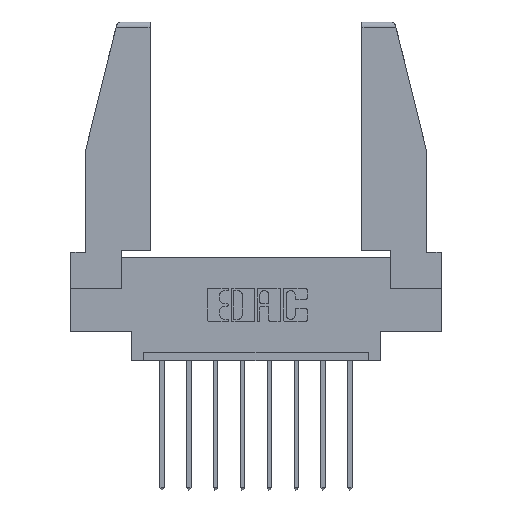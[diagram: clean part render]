
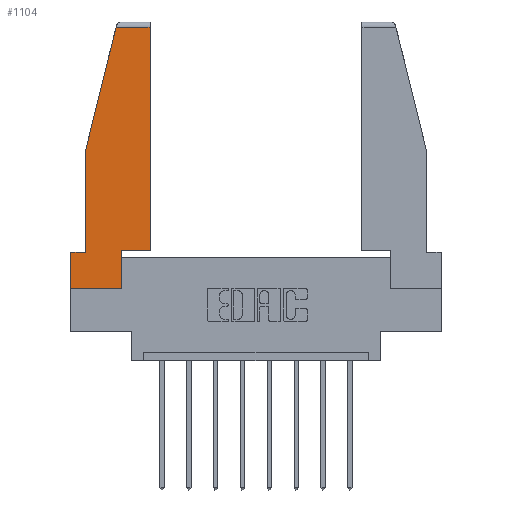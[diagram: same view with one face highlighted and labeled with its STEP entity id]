
A CAD part, top view. The second image highlights one B-rep face of the part: STEP entity #1104.
In plain terms, the highlighted planar face has unit normal (0, 0, 1).
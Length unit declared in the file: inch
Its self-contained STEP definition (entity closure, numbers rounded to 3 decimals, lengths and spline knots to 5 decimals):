
#374 = ORIENTED_EDGE ( 'NONE', *, *, #4284, .T. ) ;
#571 = CARTESIAN_POINT ( 'NONE',  ( 0.297, 0., 0. ) ) ;
#787 = VERTEX_POINT ( 'NONE', #571 ) ;
#993 = CARTESIAN_POINT ( 'NONE',  ( 0.086, 0.21, 0. ) ) ;
#1021 = VERTEX_POINT ( 'NONE', #4981 ) ;
#1044 = CARTESIAN_POINT ( 'NONE',  ( 0.297, 0.223, 0. ) ) ;
#1104 = ADVANCED_FACE ( 'NONE', ( #7009 ), #9016, .T. ) ;
#1196 = DIRECTION ( 'NONE',  ( 1., 0., 0. ) ) ;
#1366 = VERTEX_POINT ( 'NONE', #2493 ) ;
#1402 = EDGE_CURVE ( 'NONE', #1366, #1021, #10311, .T. ) ;
#1711 = ORIENTED_EDGE ( 'NONE', *, *, #8019, .T. ) ;
#1864 = LINE ( 'NONE', #9884, #8875 ) ;
#2055 = CARTESIAN_POINT ( 'NONE',  ( 0.297, 0.223, 0. ) ) ;
#2300 = LINE ( 'NONE', #12839, #4315 ) ;
#2321 = VECTOR ( 'NONE', #5635, 39.37008 ) ;
#2493 = CARTESIAN_POINT ( 'NONE',  ( 0.461, 1.52, 0. ) ) ;
#2699 = CARTESIAN_POINT ( 'NONE',  ( 0., 1.52, 0. ) ) ;
#2804 = LINE ( 'NONE', #8378, #10902 ) ;
#3089 = DIRECTION ( 'NONE',  ( 0., 0., 1. ) ) ;
#3098 = ORIENTED_EDGE ( 'NONE', *, *, #11533, .T. ) ;
#3174 = DIRECTION ( 'NONE',  ( -0.239, -0.971, 0. ) ) ;
#3208 = CARTESIAN_POINT ( 'NONE',  ( 0., 0., 0. ) ) ;
#3482 = VECTOR ( 'NONE', #10909, 39.37008 ) ;
#3798 = CARTESIAN_POINT ( 'NONE',  ( 0.086, 0.8, 0. ) ) ;
#3975 = LINE ( 'NONE', #8621, #11837 ) ;
#4070 = CARTESIAN_POINT ( 'NONE',  ( 0., 0., 0. ) ) ;
#4145 = CARTESIAN_POINT ( 'NONE',  ( 0., 0.21, 0. ) ) ;
#4284 = EDGE_CURVE ( 'NONE', #11437, #12099, #7733, .T. ) ;
#4315 = VECTOR ( 'NONE', #11836, 39.37008 ) ;
#4981 = CARTESIAN_POINT ( 'NONE',  ( 0.2636, 1.52, 0. ) ) ;
#5076 = ORIENTED_EDGE ( 'NONE', *, *, #8603, .T. ) ;
#5110 = ORIENTED_EDGE ( 'NONE', *, *, #1402, .T. ) ;
#5635 = DIRECTION ( 'NONE',  ( -1., 0., 0. ) ) ;
#5682 = EDGE_CURVE ( 'NONE', #11291, #787, #7548, .T. ) ;
#5814 = LINE ( 'NONE', #9106, #8008 ) ;
#5994 = VECTOR ( 'NONE', #11102, 39.37008 ) ;
#6063 = EDGE_CURVE ( 'NONE', #787, #7178, #5814, .T. ) ;
#6149 = EDGE_CURVE ( 'NONE', #7178, #9299, #7037, .T. ) ;
#6371 = ORIENTED_EDGE ( 'NONE', *, *, #6063, .T. ) ;
#6395 = CARTESIAN_POINT ( 'NONE',  ( 0.461, 0.223, 0. ) ) ;
#6907 = DIRECTION ( 'NONE',  ( 0., 1., 0. ) ) ;
#7009 = FACE_OUTER_BOUND ( 'NONE', #10683, .T. ) ;
#7037 = LINE ( 'NONE', #1044, #12554 ) ;
#7149 = CARTESIAN_POINT ( 'NONE',  ( 0.086, 0.8, 0. ) ) ;
#7178 = VERTEX_POINT ( 'NONE', #2055 ) ;
#7278 = ORIENTED_EDGE ( 'NONE', *, *, #9444, .T. ) ;
#7437 = VERTEX_POINT ( 'NONE', #4145 ) ;
#7548 = LINE ( 'NONE', #4070, #5994 ) ;
#7733 = LINE ( 'NONE', #3798, #3482 ) ;
#8008 = VECTOR ( 'NONE', #6907, 39.37008 ) ;
#8019 = EDGE_CURVE ( 'NONE', #1021, #11437, #1864, .T. ) ;
#8378 = CARTESIAN_POINT ( 'NONE',  ( 0., 0.21, 0. ) ) ;
#8603 = EDGE_CURVE ( 'NONE', #9299, #1366, #2300, .T. ) ;
#8621 = CARTESIAN_POINT ( 'NONE',  ( 0., 0.21, 0. ) ) ;
#8875 = VECTOR ( 'NONE', #3174, 39.37008 ) ;
#9016 = PLANE ( 'NONE',  #11665 ) ;
#9106 = CARTESIAN_POINT ( 'NONE',  ( 0.297, 0., 0. ) ) ;
#9299 = VERTEX_POINT ( 'NONE', #6395 ) ;
#9443 = DIRECTION ( 'NONE',  ( 0., -1., 0. ) ) ;
#9444 = EDGE_CURVE ( 'NONE', #12099, #7437, #3975, .T. ) ;
#9686 = DIRECTION ( 'NONE',  ( -1., 0., 0. ) ) ;
#9884 = CARTESIAN_POINT ( 'NONE',  ( 0.271, 1.55, 0. ) ) ;
#10311 = LINE ( 'NONE', #2699, #2321 ) ;
#10683 = EDGE_LOOP ( 'NONE', ( #5076, #5110, #1711, #374, #7278, #3098, #11795, #6371, #12074 ) ) ;
#10902 = VECTOR ( 'NONE', #9443, 39.37008 ) ;
#10909 = DIRECTION ( 'NONE',  ( 0., -1., 0. ) ) ;
#11091 = CARTESIAN_POINT ( 'NONE',  ( 0., 0., 0. ) ) ;
#11102 = DIRECTION ( 'NONE',  ( 1., 0., 0. ) ) ;
#11291 = VERTEX_POINT ( 'NONE', #3208 ) ;
#11437 = VERTEX_POINT ( 'NONE', #7149 ) ;
#11533 = EDGE_CURVE ( 'NONE', #7437, #11291, #2804, .T. ) ;
#11665 = AXIS2_PLACEMENT_3D ( 'NONE', #11091, #3089, #1196 ) ;
#11795 = ORIENTED_EDGE ( 'NONE', *, *, #5682, .T. ) ;
#11836 = DIRECTION ( 'NONE',  ( 0., 1., 0. ) ) ;
#11837 = VECTOR ( 'NONE', #9686, 39.37008 ) ;
#12074 = ORIENTED_EDGE ( 'NONE', *, *, #6149, .T. ) ;
#12099 = VERTEX_POINT ( 'NONE', #993 ) ;
#12554 = VECTOR ( 'NONE', #12860, 39.37008 ) ;
#12839 = CARTESIAN_POINT ( 'NONE',  ( 0.461, 0.223, 0. ) ) ;
#12860 = DIRECTION ( 'NONE',  ( 1., 0., 0. ) ) ;
